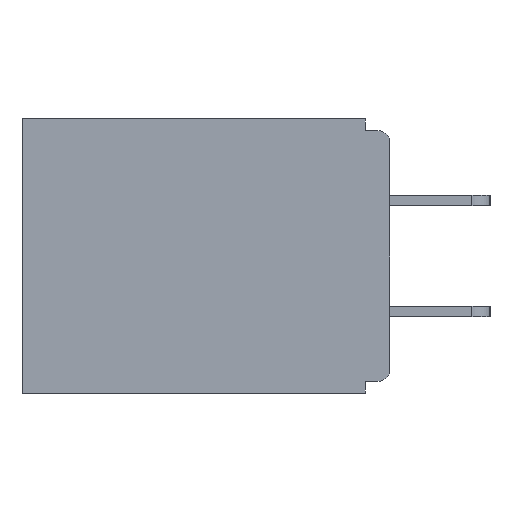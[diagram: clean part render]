
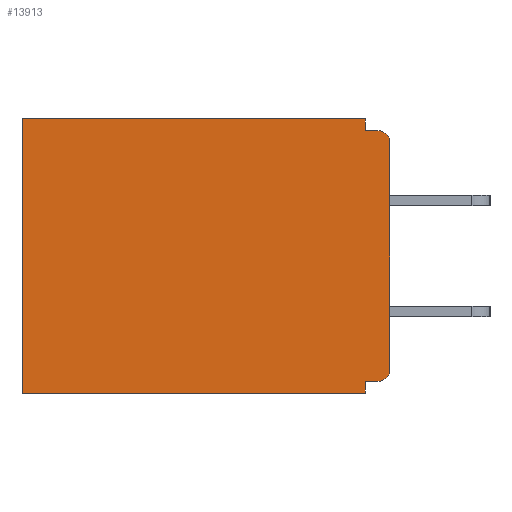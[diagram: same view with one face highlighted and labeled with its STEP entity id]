
A CAD part, left-side view. The second image highlights one B-rep face of the part: STEP entity #13913.
In plain terms, the highlighted planar face has unit normal (-1, 0, 0).
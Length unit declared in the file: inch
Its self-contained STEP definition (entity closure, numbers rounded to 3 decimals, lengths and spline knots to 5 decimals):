
#459 = CARTESIAN_POINT ( 'NONE',  ( 0.298, 0.46, -0.343 ) ) ;
#711 = CARTESIAN_POINT ( 'NONE',  ( 0.298, 0.031, -0.343 ) ) ;
#955 = LINE ( 'NONE', #16821, #17765 ) ;
#1151 = ORIENTED_EDGE ( 'NONE', *, *, #13613, .F. ) ;
#1515 = EDGE_LOOP ( 'NONE', ( #20820, #20237, #8119, #15318, #17763, #26215, #1151, #22055, #20960, #19147 ) ) ;
#1531 = CIRCLE ( 'NONE', #23082, 0.015 ) ;
#2733 = DIRECTION ( 'NONE',  ( 0., 0., -1. ) ) ;
#2819 = LINE ( 'NONE', #23420, #9264 ) ;
#2847 = CARTESIAN_POINT ( 'NONE',  ( 0.298, 0., -0.313 ) ) ;
#3416 = EDGE_CURVE ( 'NONE', #3550, #15985, #955, .T. ) ;
#3475 = DIRECTION ( 'NONE',  ( 1., 0., 0. ) ) ;
#3550 = VERTEX_POINT ( 'NONE', #24903 ) ;
#3580 = DIRECTION ( 'NONE',  ( 0., 0., -1. ) ) ;
#3838 = DIRECTION ( 'NONE',  ( 0., 1., 0. ) ) ;
#4167 = VERTEX_POINT ( 'NONE', #13350 ) ;
#4706 = VECTOR ( 'NONE', #25308, 39.37008 ) ;
#4717 = VERTEX_POINT ( 'NONE', #2847 ) ;
#4734 = LINE ( 'NONE', #10823, #4706 ) ;
#4963 = DIRECTION ( 'NONE',  ( -1., 0., 0. ) ) ;
#6441 = LINE ( 'NONE', #711, #26550 ) ;
#7384 = EDGE_CURVE ( 'NONE', #26311, #23564, #1531, .T. ) ;
#7486 = EDGE_CURVE ( 'NONE', #19639, #23197, #21595, .T. ) ;
#7521 = CARTESIAN_POINT ( 'NONE',  ( 0.298, 0., 0. ) ) ;
#7969 = VECTOR ( 'NONE', #3838, 39.37008 ) ;
#8119 = ORIENTED_EDGE ( 'NONE', *, *, #26053, .F. ) ;
#8581 = DIRECTION ( 'NONE',  ( 0., 1., 0. ) ) ;
#8915 = DIRECTION ( 'NONE',  ( 0., 0., -1. ) ) ;
#9264 = VECTOR ( 'NONE', #25522, 39.37008 ) ;
#9314 = FACE_OUTER_BOUND ( 'NONE', #1515, .T. ) ;
#9719 = DIRECTION ( 'NONE',  ( 0., 0., -1. ) ) ;
#10558 = CIRCLE ( 'NONE', #20899, 0.015 ) ;
#10823 = CARTESIAN_POINT ( 'NONE',  ( 0.298, 0., 0. ) ) ;
#11038 = LINE ( 'NONE', #21155, #14607 ) ;
#11318 = CARTESIAN_POINT ( 'NONE',  ( 0.298, 0.46, 0. ) ) ;
#11479 = VECTOR ( 'NONE', #13272, 39.37008 ) ;
#11518 = CARTESIAN_POINT ( 'NONE',  ( 0.298, 0., -0.343 ) ) ;
#13272 = DIRECTION ( 'NONE',  ( 0., 0., -1. ) ) ;
#13350 = CARTESIAN_POINT ( 'NONE',  ( 0.298, 0.031, -0.328 ) ) ;
#13613 = EDGE_CURVE ( 'NONE', #4167, #19639, #6441, .T. ) ;
#13894 = CARTESIAN_POINT ( 'NONE',  ( 0.298, 0.015, -0.03 ) ) ;
#13913 = ADVANCED_FACE ( 'NONE', ( #9314 ), #22129, .F. ) ;
#14607 = VECTOR ( 'NONE', #21248, 39.37008 ) ;
#14764 = EDGE_CURVE ( 'NONE', #26311, #4717, #4734, .T. ) ;
#14928 = VERTEX_POINT ( 'NONE', #19359 ) ;
#15044 = EDGE_CURVE ( 'NONE', #15204, #4167, #2819, .T. ) ;
#15204 = VERTEX_POINT ( 'NONE', #15551 ) ;
#15318 = ORIENTED_EDGE ( 'NONE', *, *, #3416, .T. ) ;
#15551 = CARTESIAN_POINT ( 'NONE',  ( 0.298, 0.015, -0.328 ) ) ;
#15817 = CARTESIAN_POINT ( 'NONE',  ( 0.298, 0.015, -0.015 ) ) ;
#15985 = VERTEX_POINT ( 'NONE', #19292 ) ;
#16297 = CARTESIAN_POINT ( 'NONE',  ( 0.298, 0.031, -0.343 ) ) ;
#16821 = CARTESIAN_POINT ( 'NONE',  ( 0.298, 0., 0. ) ) ;
#17377 = CARTESIAN_POINT ( 'NONE',  ( 0.298, 0.015, -0.313 ) ) ;
#17519 = EDGE_CURVE ( 'NONE', #15985, #23197, #23699, .T. ) ;
#17763 = ORIENTED_EDGE ( 'NONE', *, *, #17519, .T. ) ;
#17765 = VECTOR ( 'NONE', #8581, 39.37008 ) ;
#17856 = DIRECTION ( 'NONE',  ( -1., 0., 0. ) ) ;
#18235 = VECTOR ( 'NONE', #2733, 39.37008 ) ;
#18435 = EDGE_CURVE ( 'NONE', #14928, #23564, #11038, .T. ) ;
#19147 = ORIENTED_EDGE ( 'NONE', *, *, #14764, .F. ) ;
#19242 = LINE ( 'NONE', #25939, #11479 ) ;
#19292 = CARTESIAN_POINT ( 'NONE',  ( 0.298, 0.46, 0. ) ) ;
#19359 = CARTESIAN_POINT ( 'NONE',  ( 0.298, 0.031, -0.015 ) ) ;
#19458 = DIRECTION ( 'NONE',  ( 0., 0., -1. ) ) ;
#19639 = VERTEX_POINT ( 'NONE', #16297 ) ;
#20237 = ORIENTED_EDGE ( 'NONE', *, *, #18435, .F. ) ;
#20820 = ORIENTED_EDGE ( 'NONE', *, *, #7384, .T. ) ;
#20899 = AXIS2_PLACEMENT_3D ( 'NONE', #17377, #4963, #19458 ) ;
#20960 = ORIENTED_EDGE ( 'NONE', *, *, #24188, .T. ) ;
#21155 = CARTESIAN_POINT ( 'NONE',  ( 0.298, 0., -0.015 ) ) ;
#21248 = DIRECTION ( 'NONE',  ( 0., -1., 0. ) ) ;
#21595 = LINE ( 'NONE', #11518, #7969 ) ;
#22055 = ORIENTED_EDGE ( 'NONE', *, *, #15044, .F. ) ;
#22129 = PLANE ( 'NONE',  #22362 ) ;
#22362 = AXIS2_PLACEMENT_3D ( 'NONE', #7521, #3475, #9719 ) ;
#23082 = AXIS2_PLACEMENT_3D ( 'NONE', #13894, #17856, #3580 ) ;
#23197 = VERTEX_POINT ( 'NONE', #459 ) ;
#23420 = CARTESIAN_POINT ( 'NONE',  ( 0.298, 0., -0.328 ) ) ;
#23564 = VERTEX_POINT ( 'NONE', #15817 ) ;
#23699 = LINE ( 'NONE', #11318, #18235 ) ;
#24188 = EDGE_CURVE ( 'NONE', #15204, #4717, #10558, .T. ) ;
#24681 = CARTESIAN_POINT ( 'NONE',  ( 0.298, 0., -0.03 ) ) ;
#24903 = CARTESIAN_POINT ( 'NONE',  ( 0.298, 0.031, 0. ) ) ;
#25308 = DIRECTION ( 'NONE',  ( 0., 0., -1. ) ) ;
#25522 = DIRECTION ( 'NONE',  ( 0., 1., 0. ) ) ;
#25939 = CARTESIAN_POINT ( 'NONE',  ( 0.298, 0.031, -0.343 ) ) ;
#26053 = EDGE_CURVE ( 'NONE', #3550, #14928, #19242, .T. ) ;
#26215 = ORIENTED_EDGE ( 'NONE', *, *, #7486, .F. ) ;
#26311 = VERTEX_POINT ( 'NONE', #24681 ) ;
#26550 = VECTOR ( 'NONE', #8915, 39.37008 ) ;
